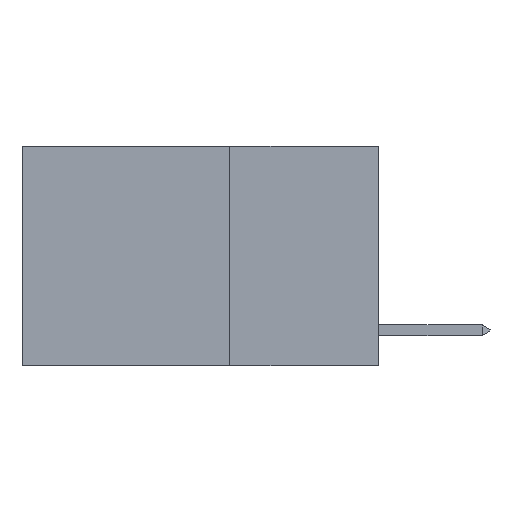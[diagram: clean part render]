
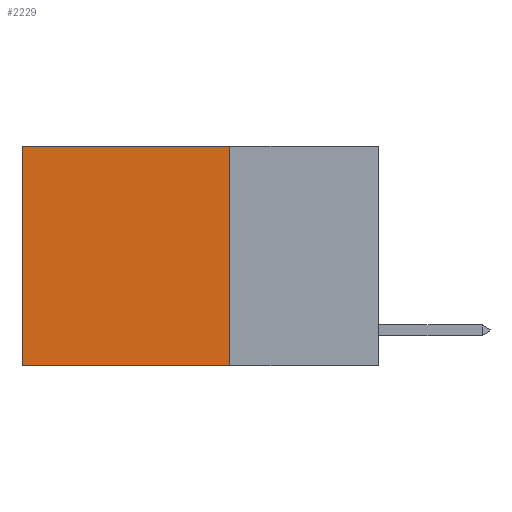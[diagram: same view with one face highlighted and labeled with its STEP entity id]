
A CAD part, left-side view. The second image highlights one B-rep face of the part: STEP entity #2229.
In plain terms, the highlighted planar face has unit normal (-1, 0, 0).
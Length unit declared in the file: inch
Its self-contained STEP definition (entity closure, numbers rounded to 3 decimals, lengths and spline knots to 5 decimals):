
#33 = LINE ( 'NONE', #4715, #2585 ) ;
#87 = CARTESIAN_POINT ( 'NONE',  ( 0.2625, 0.6, 0. ) ) ;
#241 = LINE ( 'NONE', #13442, #4424 ) ;
#530 = ORIENTED_EDGE ( 'NONE', *, *, #5173, .T. ) ;
#542 = CARTESIAN_POINT ( 'NONE',  ( 0.2625, 0.25, 0. ) ) ;
#2229 = ADVANCED_FACE ( 'NONE', ( #15121 ), #11636, .F. ) ;
#2585 = VECTOR ( 'NONE', #11145, 39.37008 ) ;
#2979 = DIRECTION ( 'NONE',  ( 0., 1., 0. ) ) ;
#4424 = VECTOR ( 'NONE', #11756, 39.37008 ) ;
#4431 = VERTEX_POINT ( 'NONE', #10228 ) ;
#4496 = DIRECTION ( 'NONE',  ( 0., 1., 0. ) ) ;
#4715 = CARTESIAN_POINT ( 'NONE',  ( 0.2625, 0.25, 0. ) ) ;
#5173 = EDGE_CURVE ( 'NONE', #14308, #20564, #241, .T. ) ;
#5645 = DIRECTION ( 'NONE',  ( 0., 0., -1. ) ) ;
#6273 = ORIENTED_EDGE ( 'NONE', *, *, #14326, .F. ) ;
#6888 = EDGE_CURVE ( 'NONE', #10451, #14308, #14199, .T. ) ;
#7268 = EDGE_LOOP ( 'NONE', ( #530, #6273, #11799, #7956 ) ) ;
#7447 = CARTESIAN_POINT ( 'NONE',  ( 0.2625, 0.25, 0. ) ) ;
#7956 = ORIENTED_EDGE ( 'NONE', *, *, #6888, .T. ) ;
#9106 = VECTOR ( 'NONE', #2979, 39.37008 ) ;
#9170 = VECTOR ( 'NONE', #4496, 39.37008 ) ;
#10228 = CARTESIAN_POINT ( 'NONE',  ( 0.2625, 0.25, -0.37 ) ) ;
#10451 = VERTEX_POINT ( 'NONE', #10882 ) ;
#10491 = DIRECTION ( 'NONE',  ( 1., 0., 0. ) ) ;
#10882 = CARTESIAN_POINT ( 'NONE',  ( 0.2625, 0.25, 0. ) ) ;
#11145 = DIRECTION ( 'NONE',  ( 0., 0., -1. ) ) ;
#11636 = PLANE ( 'NONE',  #16467 ) ;
#11756 = DIRECTION ( 'NONE',  ( 0., 0., -1. ) ) ;
#11799 = ORIENTED_EDGE ( 'NONE', *, *, #18858, .F. ) ;
#13442 = CARTESIAN_POINT ( 'NONE',  ( 0.2625, 0.6, 0. ) ) ;
#14199 = LINE ( 'NONE', #7447, #9170 ) ;
#14308 = VERTEX_POINT ( 'NONE', #87 ) ;
#14326 = EDGE_CURVE ( 'NONE', #4431, #20564, #17403, .T. ) ;
#15121 = FACE_OUTER_BOUND ( 'NONE', #7268, .T. ) ;
#15142 = CARTESIAN_POINT ( 'NONE',  ( 0.2625, 0.6, -0.37 ) ) ;
#16467 = AXIS2_PLACEMENT_3D ( 'NONE', #542, #10491, #5645 ) ;
#17403 = LINE ( 'NONE', #20672, #9106 ) ;
#18858 = EDGE_CURVE ( 'NONE', #10451, #4431, #33, .T. ) ;
#20564 = VERTEX_POINT ( 'NONE', #15142 ) ;
#20672 = CARTESIAN_POINT ( 'NONE',  ( 0.2625, 0.25, -0.37 ) ) ;
